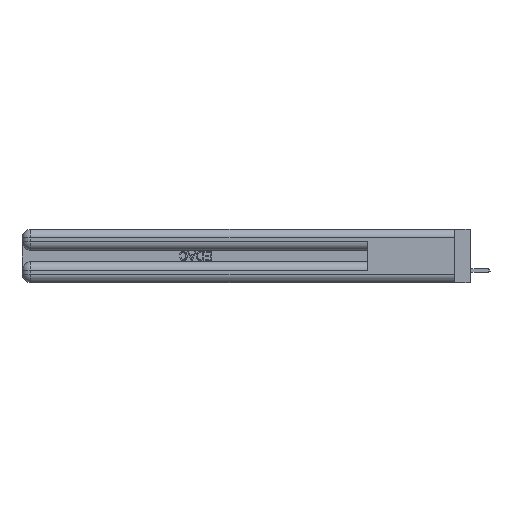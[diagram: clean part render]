
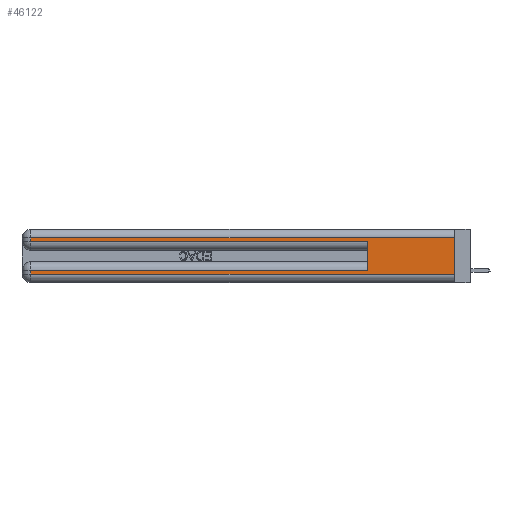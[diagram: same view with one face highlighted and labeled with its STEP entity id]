
A CAD part, left-side view. The second image highlights one B-rep face of the part: STEP entity #46122.
In plain terms, the highlighted planar face has unit normal (-1, 0, 0).
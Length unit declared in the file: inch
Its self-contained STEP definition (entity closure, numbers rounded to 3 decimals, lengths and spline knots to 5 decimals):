
#436 = CARTESIAN_POINT ( 'NONE',  ( 0., 0.6, 0.285 ) ) ;
#1163 = VECTOR ( 'NONE', #49661, 39.37008 ) ;
#2669 = LINE ( 'NONE', #5919, #33112 ) ;
#3020 = DIRECTION ( 'NONE',  ( 0., -1., 0. ) ) ;
#3824 = DIRECTION ( 'NONE',  ( 0., 1., 0. ) ) ;
#4766 = DIRECTION ( 'NONE',  ( 0., 0., -1. ) ) ;
#5892 = VECTOR ( 'NONE', #36402, 39.37008 ) ;
#5896 = VERTEX_POINT ( 'NONE', #15757 ) ;
#5919 = CARTESIAN_POINT ( 'NONE',  ( 0., 0., 0.285 ) ) ;
#8014 = EDGE_CURVE ( 'NONE', #25477, #20289, #11562, .T. ) ;
#8861 = PLANE ( 'NONE',  #46996 ) ;
#9220 = EDGE_CURVE ( 'NONE', #9612, #19118, #11393, .T. ) ;
#9612 = VERTEX_POINT ( 'NONE', #27533 ) ;
#11352 = EDGE_CURVE ( 'NONE', #16952, #25477, #34764, .T. ) ;
#11393 = LINE ( 'NONE', #15285, #48395 ) ;
#11562 = LINE ( 'NONE', #22849, #46625 ) ;
#12347 = CARTESIAN_POINT ( 'NONE',  ( 0., 0.6, 0.145 ) ) ;
#13109 = CARTESIAN_POINT ( 'NONE',  ( 0., 0., 0.37 ) ) ;
#13215 = CARTESIAN_POINT ( 'NONE',  ( 0., 0., 0.06 ) ) ;
#15285 = CARTESIAN_POINT ( 'NONE',  ( 0., 0., 0.06 ) ) ;
#15700 = ORIENTED_EDGE ( 'NONE', *, *, #9220, .T. ) ;
#15757 = CARTESIAN_POINT ( 'NONE',  ( 0., 0.6, 0.085 ) ) ;
#16292 = LINE ( 'NONE', #35120, #53291 ) ;
#16952 = VERTEX_POINT ( 'NONE', #52498 ) ;
#17816 = EDGE_CURVE ( 'NONE', #20289, #24930, #2669, .T. ) ;
#19118 = VERTEX_POINT ( 'NONE', #13215 ) ;
#19388 = CARTESIAN_POINT ( 'NONE',  ( 0., 0., 0.37 ) ) ;
#19480 = ORIENTED_EDGE ( 'NONE', *, *, #11352, .T. ) ;
#19621 = ORIENTED_EDGE ( 'NONE', *, *, #8014, .T. ) ;
#20289 = VERTEX_POINT ( 'NONE', #54317 ) ;
#21874 = EDGE_CURVE ( 'NONE', #53397, #9612, #27683, .T. ) ;
#21945 = DIRECTION ( 'NONE',  ( 1., 0., 0. ) ) ;
#22849 = CARTESIAN_POINT ( 'NONE',  ( 0., 2.94, 0.37 ) ) ;
#24930 = VERTEX_POINT ( 'NONE', #436 ) ;
#25477 = VERTEX_POINT ( 'NONE', #30724 ) ;
#25720 = LINE ( 'NONE', #19388, #5892 ) ;
#27204 = DIRECTION ( 'NONE',  ( 0., 1., 0. ) ) ;
#27533 = CARTESIAN_POINT ( 'NONE',  ( 0., 2.94, 0.06 ) ) ;
#27683 = LINE ( 'NONE', #44419, #49579 ) ;
#28100 = DIRECTION ( 'NONE',  ( 0., -1., 0. ) ) ;
#29966 = ORIENTED_EDGE ( 'NONE', *, *, #17816, .T. ) ;
#30724 = CARTESIAN_POINT ( 'NONE',  ( 0., 2.94, 0.31 ) ) ;
#31331 = EDGE_CURVE ( 'NONE', #5896, #24930, #31623, .T. ) ;
#31623 = LINE ( 'NONE', #12347, #1163 ) ;
#31724 = DIRECTION ( 'NONE',  ( 0., 0., -1. ) ) ;
#33112 = VECTOR ( 'NONE', #28100, 39.37008 ) ;
#34764 = LINE ( 'NONE', #37510, #44823 ) ;
#35120 = CARTESIAN_POINT ( 'NONE',  ( 0., 0., 0.085 ) ) ;
#35786 = EDGE_LOOP ( 'NONE', ( #45888, #19480, #19621, #29966, #44441, #43160, #44849, #15700 ) ) ;
#36257 = EDGE_CURVE ( 'NONE', #16952, #19118, #25720, .T. ) ;
#36402 = DIRECTION ( 'NONE',  ( 0., 0., -1. ) ) ;
#37510 = CARTESIAN_POINT ( 'NONE',  ( 0., 0., 0.31 ) ) ;
#39249 = EDGE_CURVE ( 'NONE', #5896, #53397, #16292, .T. ) ;
#41574 = FACE_OUTER_BOUND ( 'NONE', #35786, .T. ) ;
#43160 = ORIENTED_EDGE ( 'NONE', *, *, #39249, .T. ) ;
#44419 = CARTESIAN_POINT ( 'NONE',  ( 0., 2.94, 0.37 ) ) ;
#44441 = ORIENTED_EDGE ( 'NONE', *, *, #31331, .F. ) ;
#44823 = VECTOR ( 'NONE', #3824, 39.37008 ) ;
#44849 = ORIENTED_EDGE ( 'NONE', *, *, #21874, .T. ) ;
#45888 = ORIENTED_EDGE ( 'NONE', *, *, #36257, .F. ) ;
#46122 = ADVANCED_FACE ( 'NONE', ( #41574 ), #8861, .F. ) ;
#46625 = VECTOR ( 'NONE', #52457, 39.37008 ) ;
#46996 = AXIS2_PLACEMENT_3D ( 'NONE', #13109, #21945, #4766 ) ;
#48395 = VECTOR ( 'NONE', #3020, 39.37008 ) ;
#49579 = VECTOR ( 'NONE', #31724, 39.37008 ) ;
#49661 = DIRECTION ( 'NONE',  ( 0., 0., 1. ) ) ;
#50305 = CARTESIAN_POINT ( 'NONE',  ( 0., 2.94, 0.085 ) ) ;
#52457 = DIRECTION ( 'NONE',  ( 0., 0., -1. ) ) ;
#52498 = CARTESIAN_POINT ( 'NONE',  ( 0., 0., 0.31 ) ) ;
#53291 = VECTOR ( 'NONE', #27204, 39.37008 ) ;
#53397 = VERTEX_POINT ( 'NONE', #50305 ) ;
#54317 = CARTESIAN_POINT ( 'NONE',  ( 0., 2.94, 0.285 ) ) ;
